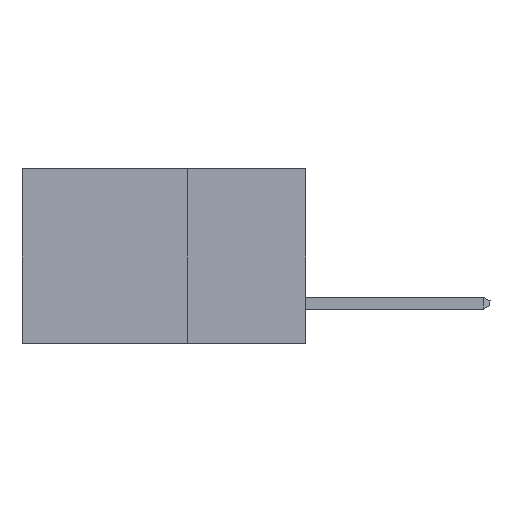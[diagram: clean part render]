
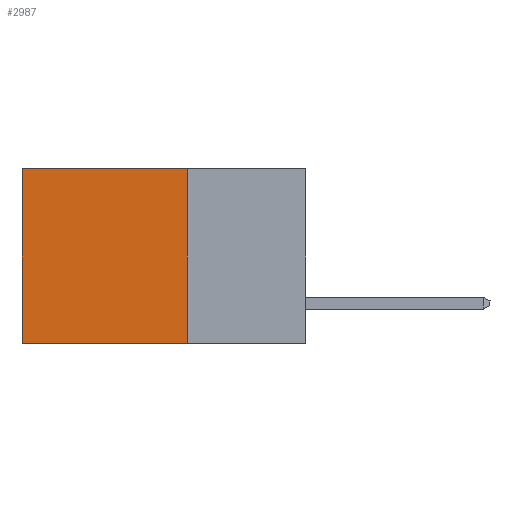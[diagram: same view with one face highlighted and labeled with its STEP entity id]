
A CAD part, left-side view. The second image highlights one B-rep face of the part: STEP entity #2987.
In plain terms, the highlighted planar face has unit normal (-1, 0, 0).
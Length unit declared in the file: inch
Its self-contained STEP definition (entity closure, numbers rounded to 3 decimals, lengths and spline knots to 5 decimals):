
#142 = ORIENTED_EDGE ( 'NONE', *, *, #2734, .T. ) ;
#483 = EDGE_CURVE ( 'NONE', #8136, #971, #8731, .T. ) ;
#550 = CARTESIAN_POINT ( 'NONE',  ( 0.2615, 0.25, -0.37 ) ) ;
#860 = CARTESIAN_POINT ( 'NONE',  ( 0.2615, 0.25, -0.37 ) ) ;
#971 = VERTEX_POINT ( 'NONE', #5840 ) ;
#1992 = FACE_OUTER_BOUND ( 'NONE', #8068, .T. ) ;
#2343 = CARTESIAN_POINT ( 'NONE',  ( 0.2615, 0.25, -0.37 ) ) ;
#2500 = EDGE_CURVE ( 'NONE', #5230, #7853, #6304, .T. ) ;
#2734 = EDGE_CURVE ( 'NONE', #7853, #971, #4633, .T. ) ;
#2987 = ADVANCED_FACE ( 'NONE', ( #1992 ), #7766, .F. ) ;
#3184 = CARTESIAN_POINT ( 'NONE',  ( 0.2615, 0.6, -0.37 ) ) ;
#4299 = CARTESIAN_POINT ( 'NONE',  ( 0.2615, 0.25, -0.37 ) ) ;
#4340 = DIRECTION ( 'NONE',  ( 0., 0., -1. ) ) ;
#4369 = CARTESIAN_POINT ( 'NONE',  ( 0.2615, 0.6, 0. ) ) ;
#4633 = LINE ( 'NONE', #3184, #5323 ) ;
#5059 = VECTOR ( 'NONE', #7793, 39.37008 ) ;
#5230 = VERTEX_POINT ( 'NONE', #7683 ) ;
#5323 = VECTOR ( 'NONE', #6152, 39.37008 ) ;
#5474 = EDGE_CURVE ( 'NONE', #5230, #8136, #8802, .T. ) ;
#5840 = CARTESIAN_POINT ( 'NONE',  ( 0.2615, 0.6, -0.37 ) ) ;
#5858 = DIRECTION ( 'NONE',  ( 0., 1., 0. ) ) ;
#5916 = VECTOR ( 'NONE', #8526, 39.37008 ) ;
#6152 = DIRECTION ( 'NONE',  ( 0., 0., -1. ) ) ;
#6304 = LINE ( 'NONE', #8425, #5916 ) ;
#6360 = ORIENTED_EDGE ( 'NONE', *, *, #483, .F. ) ;
#6716 = VECTOR ( 'NONE', #5858, 39.37008 ) ;
#7605 = ORIENTED_EDGE ( 'NONE', *, *, #2500, .T. ) ;
#7683 = CARTESIAN_POINT ( 'NONE',  ( 0.2615, 0.25, 0. ) ) ;
#7766 = PLANE ( 'NONE',  #7899 ) ;
#7793 = DIRECTION ( 'NONE',  ( 0., 0., -1. ) ) ;
#7853 = VERTEX_POINT ( 'NONE', #4369 ) ;
#7899 = AXIS2_PLACEMENT_3D ( 'NONE', #860, #8696, #4340 ) ;
#8068 = EDGE_LOOP ( 'NONE', ( #142, #6360, #8851, #7605 ) ) ;
#8136 = VERTEX_POINT ( 'NONE', #550 ) ;
#8425 = CARTESIAN_POINT ( 'NONE',  ( 0.2615, 0.25, 0. ) ) ;
#8526 = DIRECTION ( 'NONE',  ( 0., 1., 0. ) ) ;
#8696 = DIRECTION ( 'NONE',  ( 1., 0., 0. ) ) ;
#8731 = LINE ( 'NONE', #4299, #6716 ) ;
#8802 = LINE ( 'NONE', #2343, #5059 ) ;
#8851 = ORIENTED_EDGE ( 'NONE', *, *, #5474, .F. ) ;
